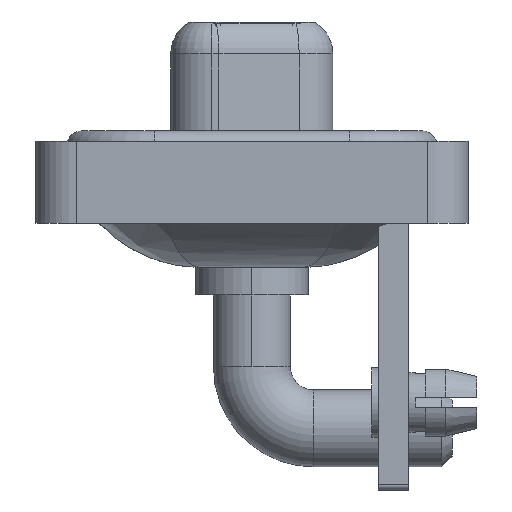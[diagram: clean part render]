
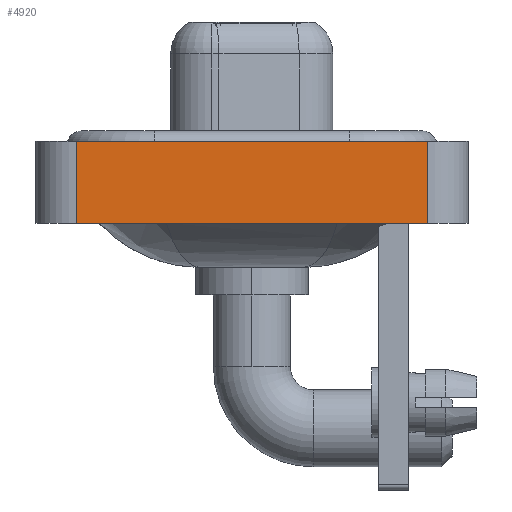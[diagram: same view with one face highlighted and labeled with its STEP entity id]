
A CAD part, left-side view. The second image highlights one B-rep face of the part: STEP entity #4920.
In plain terms, the highlighted planar face has unit normal (-1, 0, 0).
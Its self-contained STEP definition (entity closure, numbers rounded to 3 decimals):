
#305 = DIRECTION ( 'NONE',  ( 0., 0., 1. ) ) ;
#898 = EDGE_LOOP ( 'NONE', ( #4674, #17371, #5619, #16983 ) ) ;
#1957 = VERTEX_POINT ( 'NONE', #11458 ) ;
#2766 = CARTESIAN_POINT ( 'NONE',  ( -7.25, -8.55, -3.6 ) ) ;
#3093 = CARTESIAN_POINT ( 'NONE',  ( -7.25, 8.55, 0.4 ) ) ;
#3804 = CARTESIAN_POINT ( 'NONE',  ( -7.25, -8.55, -3.6 ) ) ;
#4281 = VERTEX_POINT ( 'NONE', #3093 ) ;
#4493 = EDGE_CURVE ( 'NONE', #8663, #4281, #12845, .T. ) ;
#4674 = ORIENTED_EDGE ( 'NONE', *, *, #10974, .T. ) ;
#4920 = ADVANCED_FACE ( 'NONE', ( #10230 ), #15699, .T. ) ;
#5477 = CARTESIAN_POINT ( 'NONE',  ( -7.25, -8.55, 0.4 ) ) ;
#5619 = ORIENTED_EDGE ( 'NONE', *, *, #4493, .F. ) ;
#6408 = VECTOR ( 'NONE', #7063, 1000. ) ;
#7063 = DIRECTION ( 'NONE',  ( 0., -1., 0. ) ) ;
#7500 = DIRECTION ( 'NONE',  ( 0., 0., 1. ) ) ;
#7645 = VECTOR ( 'NONE', #7500, 1000. ) ;
#8663 = VERTEX_POINT ( 'NONE', #14217 ) ;
#9449 = EDGE_CURVE ( 'NONE', #8663, #1957, #16856, .T. ) ;
#10230 = FACE_OUTER_BOUND ( 'NONE', #898, .T. ) ;
#10974 = EDGE_CURVE ( 'NONE', #1957, #12162, #12844, .T. ) ;
#11458 = CARTESIAN_POINT ( 'NONE',  ( -7.25, -8.55, -3.6 ) ) ;
#11560 = CARTESIAN_POINT ( 'NONE',  ( -7.25, 8.55, -3.6 ) ) ;
#12162 = VERTEX_POINT ( 'NONE', #12940 ) ;
#12668 = AXIS2_PLACEMENT_3D ( 'NONE', #2766, #14039, #17103 ) ;
#12844 = LINE ( 'NONE', #12937, #16965 ) ;
#12845 = LINE ( 'NONE', #11560, #7645 ) ;
#12937 = CARTESIAN_POINT ( 'NONE',  ( -7.25, -8.55, -3.6 ) ) ;
#12940 = CARTESIAN_POINT ( 'NONE',  ( -7.25, -8.55, 0.4 ) ) ;
#14039 = DIRECTION ( 'NONE',  ( -1., 0., 0. ) ) ;
#14154 = LINE ( 'NONE', #5477, #6408 ) ;
#14217 = CARTESIAN_POINT ( 'NONE',  ( -7.25, 8.55, -3.6 ) ) ;
#15448 = DIRECTION ( 'NONE',  ( 0., -1., 0. ) ) ;
#15699 = PLANE ( 'NONE',  #12668 ) ;
#16708 = VECTOR ( 'NONE', #15448, 1000. ) ;
#16856 = LINE ( 'NONE', #3804, #16708 ) ;
#16965 = VECTOR ( 'NONE', #305, 1000. ) ;
#16983 = ORIENTED_EDGE ( 'NONE', *, *, #9449, .T. ) ;
#17103 = DIRECTION ( 'NONE',  ( 0., 0., 1. ) ) ;
#17371 = ORIENTED_EDGE ( 'NONE', *, *, #18020, .F. ) ;
#18020 = EDGE_CURVE ( 'NONE', #4281, #12162, #14154, .T. ) ;
